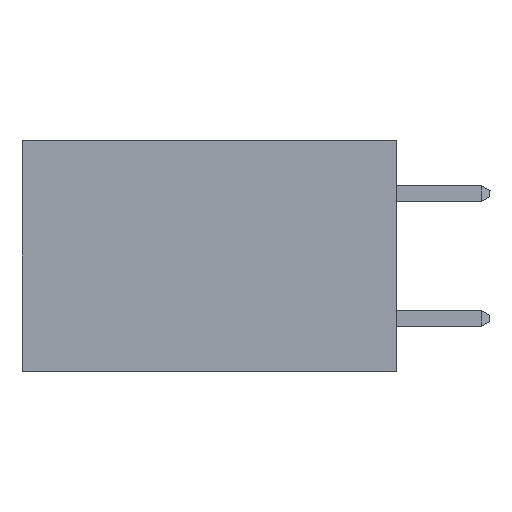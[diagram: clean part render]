
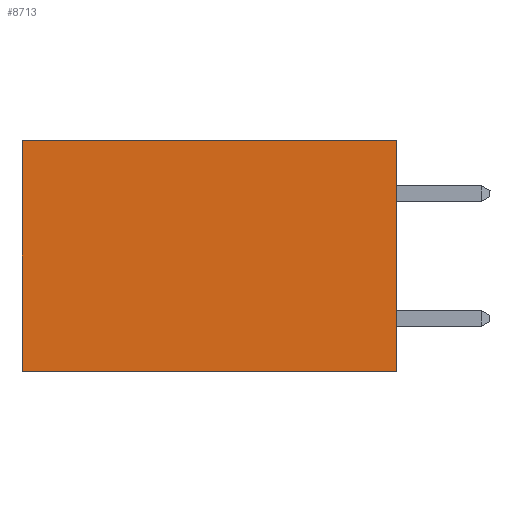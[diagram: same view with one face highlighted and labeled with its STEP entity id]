
A CAD part, left-side view. The second image highlights one B-rep face of the part: STEP entity #8713.
In plain terms, the highlighted planar face has unit normal (-1, 0, 0).
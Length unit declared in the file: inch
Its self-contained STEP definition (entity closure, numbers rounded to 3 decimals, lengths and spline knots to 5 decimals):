
#565 = EDGE_CURVE ( 'NONE', #1200, #11958, #10813, .T. ) ;
#1200 = VERTEX_POINT ( 'NONE', #3219 ) ;
#1700 = EDGE_LOOP ( 'NONE', ( #12236, #12585, #8413, #7542 ) ) ;
#2344 = DIRECTION ( 'NONE',  ( 0., 0., -1. ) ) ;
#2425 = EDGE_CURVE ( 'NONE', #4336, #1200, #6741, .T. ) ;
#2873 = VERTEX_POINT ( 'NONE', #8304 ) ;
#3091 = DIRECTION ( 'NONE',  ( 0., 1., 0. ) ) ;
#3219 = CARTESIAN_POINT ( 'NONE',  ( 0.298, 0., -0.37 ) ) ;
#3538 = CARTESIAN_POINT ( 'NONE',  ( 0.298, 0.6, 0. ) ) ;
#4183 = LINE ( 'NONE', #3538, #9891 ) ;
#4336 = VERTEX_POINT ( 'NONE', #10364 ) ;
#4505 = LINE ( 'NONE', #9619, #13356 ) ;
#4866 = CARTESIAN_POINT ( 'NONE',  ( 0.298, 0., 0. ) ) ;
#5114 = VECTOR ( 'NONE', #11085, 39.37008 ) ;
#6741 = LINE ( 'NONE', #4866, #8927 ) ;
#7136 = DIRECTION ( 'NONE',  ( 0., 0., -1. ) ) ;
#7542 = ORIENTED_EDGE ( 'NONE', *, *, #11485, .T. ) ;
#7637 = DIRECTION ( 'NONE',  ( 0., 0., -1. ) ) ;
#7653 = DIRECTION ( 'NONE',  ( 1., 0., 0. ) ) ;
#7669 = CARTESIAN_POINT ( 'NONE',  ( 0.298, 0., 0. ) ) ;
#7813 = PLANE ( 'NONE',  #12729 ) ;
#8304 = CARTESIAN_POINT ( 'NONE',  ( 0.298, 0.6, 0. ) ) ;
#8413 = ORIENTED_EDGE ( 'NONE', *, *, #2425, .F. ) ;
#8713 = ADVANCED_FACE ( 'NONE', ( #9884 ), #7813, .F. ) ;
#8927 = VECTOR ( 'NONE', #7136, 39.37008 ) ;
#9619 = CARTESIAN_POINT ( 'NONE',  ( 0.298, 0., 0. ) ) ;
#9884 = FACE_OUTER_BOUND ( 'NONE', #1700, .T. ) ;
#9891 = VECTOR ( 'NONE', #2344, 39.37008 ) ;
#10172 = CARTESIAN_POINT ( 'NONE',  ( 0.298, 0.6, -0.37 ) ) ;
#10250 = EDGE_CURVE ( 'NONE', #2873, #11958, #4183, .T. ) ;
#10364 = CARTESIAN_POINT ( 'NONE',  ( 0.298, 0., 0. ) ) ;
#10813 = LINE ( 'NONE', #14029, #5114 ) ;
#11085 = DIRECTION ( 'NONE',  ( 0., 1., 0. ) ) ;
#11485 = EDGE_CURVE ( 'NONE', #4336, #2873, #4505, .T. ) ;
#11958 = VERTEX_POINT ( 'NONE', #10172 ) ;
#12236 = ORIENTED_EDGE ( 'NONE', *, *, #10250, .T. ) ;
#12585 = ORIENTED_EDGE ( 'NONE', *, *, #565, .F. ) ;
#12729 = AXIS2_PLACEMENT_3D ( 'NONE', #7669, #7653, #7637 ) ;
#13356 = VECTOR ( 'NONE', #3091, 39.37008 ) ;
#14029 = CARTESIAN_POINT ( 'NONE',  ( 0.298, 0., -0.37 ) ) ;
